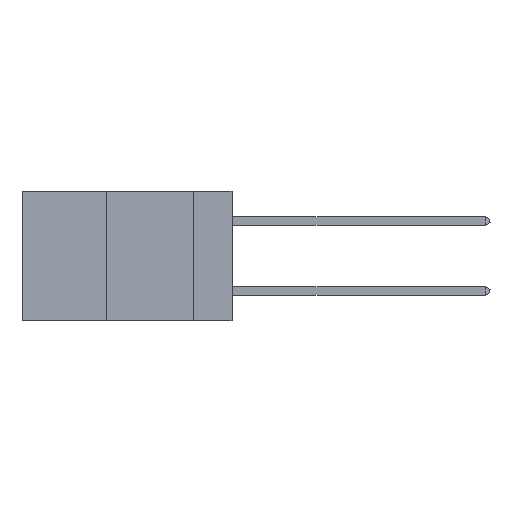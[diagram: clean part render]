
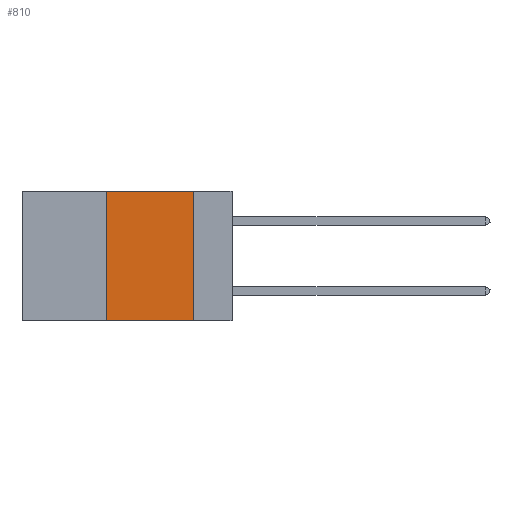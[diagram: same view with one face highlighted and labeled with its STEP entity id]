
A CAD part, left-side view. The second image highlights one B-rep face of the part: STEP entity #810.
In plain terms, the highlighted planar face has unit normal (-1, 0, 0).
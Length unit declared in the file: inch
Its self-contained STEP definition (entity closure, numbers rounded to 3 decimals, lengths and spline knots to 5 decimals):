
#810 = ADVANCED_FACE ( 'NONE', ( #12644 ), #31420, .F. ) ;
#879 = CARTESIAN_POINT ( 'NONE',  ( 0., 0.11, 0. ) ) ;
#1301 = EDGE_CURVE ( 'NONE', #31521, #11435, #30148, .T. ) ;
#3564 = DIRECTION ( 'NONE',  ( 0., -1., 0. ) ) ;
#4695 = AXIS2_PLACEMENT_3D ( 'NONE', #13393, #46092, #28093 ) ;
#5510 = ORIENTED_EDGE ( 'NONE', *, *, #1301, .F. ) ;
#5816 = CARTESIAN_POINT ( 'NONE',  ( 0., 0.36, 0. ) ) ;
#6315 = VECTOR ( 'NONE', #31329, 39.37008 ) ;
#7994 = VERTEX_POINT ( 'NONE', #11167 ) ;
#8048 = ORIENTED_EDGE ( 'NONE', *, *, #8047, .F. ) ;
#8047 = EDGE_CURVE ( 'NONE', #11435, #44222, #28201, .T. ) ;
#9852 = ORIENTED_EDGE ( 'NONE', *, *, #22180, .F. ) ;
#11167 = CARTESIAN_POINT ( 'NONE',  ( 0., 0.11, -0.37 ) ) ;
#11435 = VERTEX_POINT ( 'NONE', #5816 ) ;
#12644 = FACE_OUTER_BOUND ( 'NONE', #39585, .T. ) ;
#13393 = CARTESIAN_POINT ( 'NONE',  ( 0., 0.6, 0. ) ) ;
#14867 = DIRECTION ( 'NONE',  ( 0., -1., 0. ) ) ;
#20841 = VECTOR ( 'NONE', #3564, 39.37008 ) ;
#21386 = LINE ( 'NONE', #27195, #6315 ) ;
#22180 = EDGE_CURVE ( 'NONE', #44222, #7994, #21386, .T. ) ;
#22402 = EDGE_CURVE ( 'NONE', #31521, #7994, #45447, .T. ) ;
#22482 = ORIENTED_EDGE ( 'NONE', *, *, #22402, .T. ) ;
#27195 = CARTESIAN_POINT ( 'NONE',  ( 0., 0.11, 0. ) ) ;
#28093 = DIRECTION ( 'NONE',  ( 0., 0., -1. ) ) ;
#28201 = LINE ( 'NONE', #32930, #20841 ) ;
#28739 = DIRECTION ( 'NONE',  ( 0., 0., 1. ) ) ;
#30148 = LINE ( 'NONE', #31616, #38618 ) ;
#30726 = CARTESIAN_POINT ( 'NONE',  ( 0., 0.36, -0.37 ) ) ;
#31329 = DIRECTION ( 'NONE',  ( 0., 0., -1. ) ) ;
#31420 = PLANE ( 'NONE',  #4695 ) ;
#31521 = VERTEX_POINT ( 'NONE', #30726 ) ;
#31616 = CARTESIAN_POINT ( 'NONE',  ( 0., 0.36, 0. ) ) ;
#32930 = CARTESIAN_POINT ( 'NONE',  ( 0., 0.6, 0. ) ) ;
#38618 = VECTOR ( 'NONE', #28739, 39.37008 ) ;
#38697 = VECTOR ( 'NONE', #14867, 39.37008 ) ;
#39585 = EDGE_LOOP ( 'NONE', ( #9852, #8048, #5510, #22482 ) ) ;
#43445 = CARTESIAN_POINT ( 'NONE',  ( 0., 0.6, -0.37 ) ) ;
#44222 = VERTEX_POINT ( 'NONE', #879 ) ;
#45447 = LINE ( 'NONE', #43445, #38697 ) ;
#46092 = DIRECTION ( 'NONE',  ( 1., 0., 0. ) ) ;
